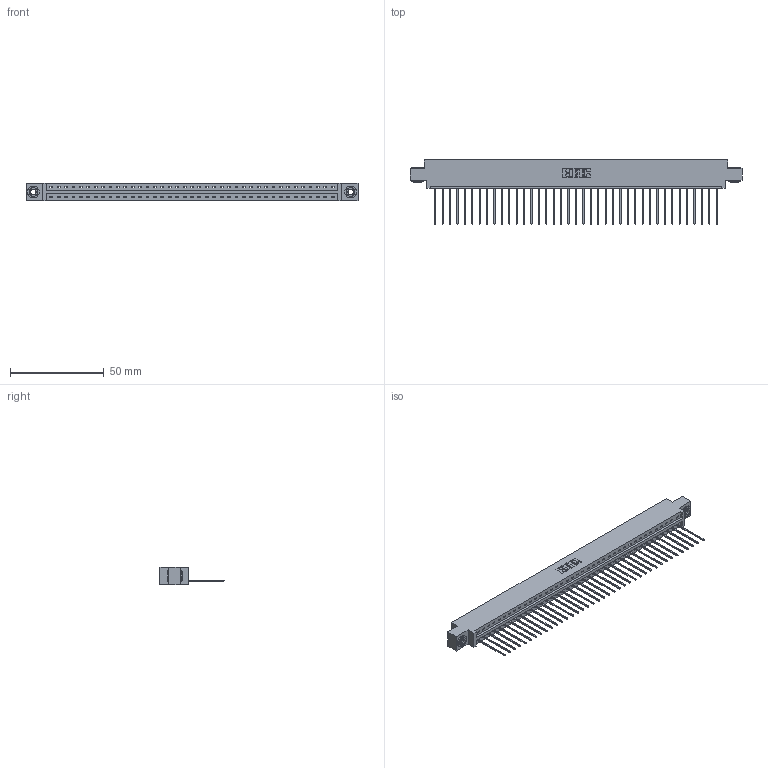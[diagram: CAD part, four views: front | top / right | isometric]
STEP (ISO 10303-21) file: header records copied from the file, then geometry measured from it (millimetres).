
FILE_DESCRIPTION (( 'STEP AP203' ), '1' );
FILE_NAME ('337-039-541-603.STEP', '2019-10-01T18:44:35', ( '' ), ( '' ), 'SwSTEP 2.0', 'SolidWorks 2016', '' );
FILE_SCHEMA (( 'CONFIG_CONTROL_DESIGN' ));
Length unit declared in the file: inch
Products named in the file (4): 345-250-002_345-250-002-102; 345-292-001_345-293-141; 337 Part_0.170 Offset - 0.156 Dia-TH; 337-039-541-603
Assembly tree (42 placements, depth 2):
  337-039-541-603
    337 Part_0.170 Offset - 0.156 Dia-TH
    345-292-001_345-293-141  x39
    345-250-002_345-250-002-102  x2
Bounding box: 177.55 x 34.3 x 9.4 mm (x, y, z)
Volume: 18446 mm3; surface area: 20165.3 mm2
Topology: 42 solids, 42 shells, 2574 faces, 7731 edges, 5098 vertices
Faces by surface type: plane 1878, cylinder 688, cone 8
Entity records: 30178 total; most frequent: CARTESIAN_POINT 5234, ORIENTED_EDGE 5202, DIRECTION 4445, EDGE_CURVE 2601, LINE 2449, VECTOR 2449, VERTEX_POINT 1730, AXIS2_PLACEMENT_3D 998
